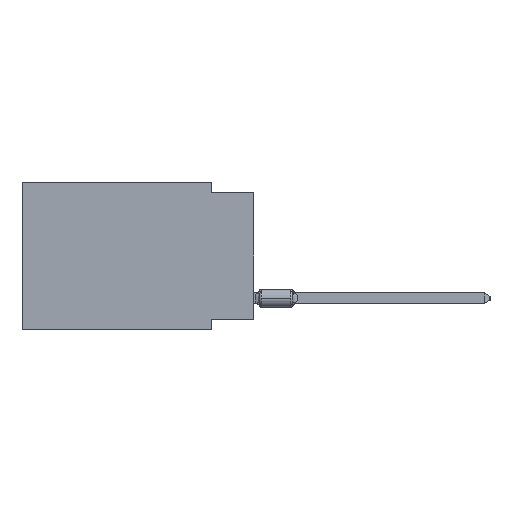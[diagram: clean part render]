
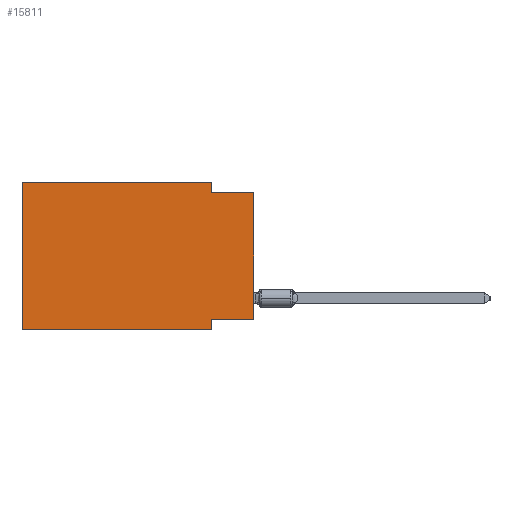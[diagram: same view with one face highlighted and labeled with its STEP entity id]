
A CAD part, left-side view. The second image highlights one B-rep face of the part: STEP entity #15811.
In plain terms, the highlighted planar face has unit normal (-1, 0, 0).
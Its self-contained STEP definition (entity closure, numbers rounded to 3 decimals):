
#332 = CARTESIAN_POINT ( 'NONE',  ( 0., 0., -0.635 ) ) ;
#702 = ORIENTED_EDGE ( 'NONE', *, *, #25406, .F. ) ;
#1743 = LINE ( 'NONE', #21761, #24978 ) ;
#3347 = DIRECTION ( 'NONE',  ( 0., -1., 0. ) ) ;
#3385 = VECTOR ( 'NONE', #10965, 1000. ) ;
#4208 = EDGE_CURVE ( 'NONE', #22607, #4903, #1743, .T. ) ;
#4903 = VERTEX_POINT ( 'NONE', #26254 ) ;
#5647 = VERTEX_POINT ( 'NONE', #332 ) ;
#6641 = VERTEX_POINT ( 'NONE', #18369 ) ;
#6745 = LINE ( 'NONE', #12938, #30111 ) ;
#6976 = ORIENTED_EDGE ( 'NONE', *, *, #19398, .F. ) ;
#7217 = VECTOR ( 'NONE', #26033, 1000. ) ;
#7563 = DIRECTION ( 'NONE',  ( 0., 0., -1. ) ) ;
#9938 = CARTESIAN_POINT ( 'NONE',  ( 0., 2.54, -8.255 ) ) ;
#10284 = VERTEX_POINT ( 'NONE', #28463 ) ;
#10717 = EDGE_CURVE ( 'NONE', #10284, #22607, #20212, .T. ) ;
#10965 = DIRECTION ( 'NONE',  ( 0., 0., 1. ) ) ;
#11044 = FACE_OUTER_BOUND ( 'NONE', #18170, .T. ) ;
#11200 = LINE ( 'NONE', #30497, #22489 ) ;
#11327 = CARTESIAN_POINT ( 'NONE',  ( 0., 13.97, 0. ) ) ;
#12548 = CARTESIAN_POINT ( 'NONE',  ( 0., 0., -8.255 ) ) ;
#12938 = CARTESIAN_POINT ( 'NONE',  ( 0., 2.54, 0. ) ) ;
#13768 = PLANE ( 'NONE',  #28597 ) ;
#14993 = VERTEX_POINT ( 'NONE', #16769 ) ;
#15371 = CARTESIAN_POINT ( 'NONE',  ( 0., 2.54, 0. ) ) ;
#15455 = DIRECTION ( 'NONE',  ( 0., -1., 0. ) ) ;
#15465 = VERTEX_POINT ( 'NONE', #33314 ) ;
#15811 = ADVANCED_FACE ( 'NONE', ( #11044 ), #13768, .F. ) ;
#16349 = LINE ( 'NONE', #27475, #31143 ) ;
#16769 = CARTESIAN_POINT ( 'NONE',  ( 0., 13.97, -8.89 ) ) ;
#18170 = EDGE_LOOP ( 'NONE', ( #19012, #27750, #702, #18367, #6976, #26780, #27758, #31696 ) ) ;
#18367 = ORIENTED_EDGE ( 'NONE', *, *, #29155, .F. ) ;
#18369 = CARTESIAN_POINT ( 'NONE',  ( 0., 2.54, -0.635 ) ) ;
#19012 = ORIENTED_EDGE ( 'NONE', *, *, #29358, .T. ) ;
#19398 = EDGE_CURVE ( 'NONE', #14993, #15465, #35904, .T. ) ;
#20212 = LINE ( 'NONE', #12548, #7217 ) ;
#20560 = LINE ( 'NONE', #21097, #26742 ) ;
#21097 = CARTESIAN_POINT ( 'NONE',  ( 0., 13.97, -8.89 ) ) ;
#21622 = DIRECTION ( 'NONE',  ( 0., 0., -1. ) ) ;
#21761 = CARTESIAN_POINT ( 'NONE',  ( 0., 2.54, -8.89 ) ) ;
#22085 = EDGE_CURVE ( 'NONE', #14993, #4903, #20560, .T. ) ;
#22489 = VECTOR ( 'NONE', #3347, 1000. ) ;
#22607 = VERTEX_POINT ( 'NONE', #9938 ) ;
#23550 = VECTOR ( 'NONE', #15455, 1000. ) ;
#23653 = CARTESIAN_POINT ( 'NONE',  ( 0., 13.97, 0. ) ) ;
#24978 = VECTOR ( 'NONE', #7563, 1000. ) ;
#25406 = EDGE_CURVE ( 'NONE', #32636, #6641, #6745, .T. ) ;
#26033 = DIRECTION ( 'NONE',  ( 0., 1., 0. ) ) ;
#26254 = CARTESIAN_POINT ( 'NONE',  ( 0., 2.54, -8.89 ) ) ;
#26461 = EDGE_CURVE ( 'NONE', #6641, #5647, #11200, .T. ) ;
#26742 = VECTOR ( 'NONE', #28764, 1000. ) ;
#26780 = ORIENTED_EDGE ( 'NONE', *, *, #22085, .T. ) ;
#27456 = CARTESIAN_POINT ( 'NONE',  ( 0., 13.97, 0. ) ) ;
#27475 = CARTESIAN_POINT ( 'NONE',  ( 0., 0., 0. ) ) ;
#27750 = ORIENTED_EDGE ( 'NONE', *, *, #26461, .F. ) ;
#27758 = ORIENTED_EDGE ( 'NONE', *, *, #4208, .F. ) ;
#28463 = CARTESIAN_POINT ( 'NONE',  ( 0., 0., -8.255 ) ) ;
#28597 = AXIS2_PLACEMENT_3D ( 'NONE', #27456, #30532, #21622 ) ;
#28764 = DIRECTION ( 'NONE',  ( 0., -1., 0. ) ) ;
#28945 = LINE ( 'NONE', #23653, #23550 ) ;
#29155 = EDGE_CURVE ( 'NONE', #15465, #32636, #28945, .T. ) ;
#29358 = EDGE_CURVE ( 'NONE', #10284, #5647, #16349, .T. ) ;
#30111 = VECTOR ( 'NONE', #31698, 1000. ) ;
#30497 = CARTESIAN_POINT ( 'NONE',  ( 0., 0., -0.635 ) ) ;
#30532 = DIRECTION ( 'NONE',  ( 1., 0., 0. ) ) ;
#31143 = VECTOR ( 'NONE', #33107, 1000. ) ;
#31696 = ORIENTED_EDGE ( 'NONE', *, *, #10717, .F. ) ;
#31698 = DIRECTION ( 'NONE',  ( 0., 0., -1. ) ) ;
#32636 = VERTEX_POINT ( 'NONE', #15371 ) ;
#33107 = DIRECTION ( 'NONE',  ( 0., 0., 1. ) ) ;
#33314 = CARTESIAN_POINT ( 'NONE',  ( 0., 13.97, 0. ) ) ;
#35904 = LINE ( 'NONE', #11327, #3385 ) ;
